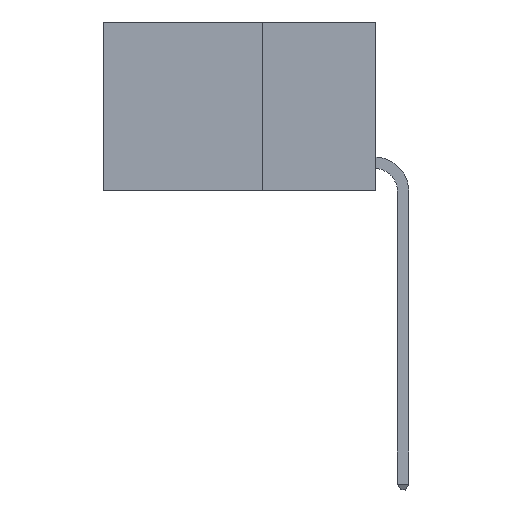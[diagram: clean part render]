
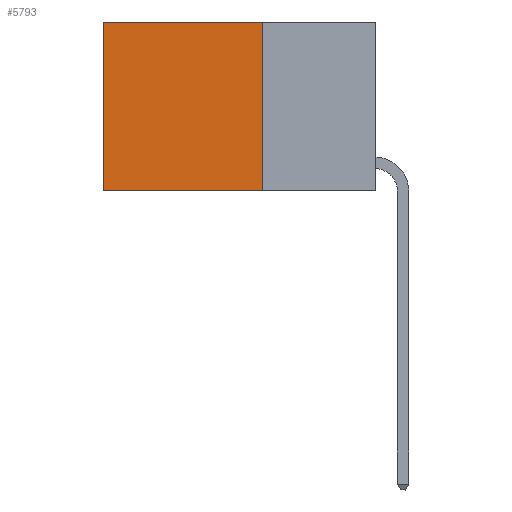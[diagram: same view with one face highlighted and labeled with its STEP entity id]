
A CAD part, left-side view. The second image highlights one B-rep face of the part: STEP entity #5793.
In plain terms, the highlighted planar face has unit normal (-1, 0, 0).
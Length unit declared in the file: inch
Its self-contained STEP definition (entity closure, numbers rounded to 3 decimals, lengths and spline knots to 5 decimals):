
#1654 = DIRECTION ( 'NONE',  ( 1., 0., 0. ) ) ;
#2324 = VERTEX_POINT ( 'NONE', #18005 ) ;
#2935 = VECTOR ( 'NONE', #12799, 39.37008 ) ;
#3043 = CARTESIAN_POINT ( 'NONE',  ( 0.2625, 0.25, 0. ) ) ;
#3224 = VECTOR ( 'NONE', #13335, 39.37008 ) ;
#5793 = ADVANCED_FACE ( 'NONE', ( #10645 ), #13223, .F. ) ;
#7062 = EDGE_CURVE ( 'NONE', #20031, #13822, #12133, .T. ) ;
#7628 = ORIENTED_EDGE ( 'NONE', *, *, #7062, .T. ) ;
#8103 = LINE ( 'NONE', #14609, #2935 ) ;
#8305 = EDGE_CURVE ( 'NONE', #20031, #17705, #24687, .T. ) ;
#8434 = ORIENTED_EDGE ( 'NONE', *, *, #9219, .T. ) ;
#8855 = ORIENTED_EDGE ( 'NONE', *, *, #16244, .F. ) ;
#8932 = DIRECTION ( 'NONE',  ( 0., 0., -1. ) ) ;
#8996 = LINE ( 'NONE', #22740, #3224 ) ;
#9219 = EDGE_CURVE ( 'NONE', #13822, #2324, #8996, .T. ) ;
#10230 = VECTOR ( 'NONE', #8932, 39.37008 ) ;
#10645 = FACE_OUTER_BOUND ( 'NONE', #12396, .T. ) ;
#12133 = LINE ( 'NONE', #3043, #22196 ) ;
#12396 = EDGE_LOOP ( 'NONE', ( #8434, #8855, #18407, #7628 ) ) ;
#12799 = DIRECTION ( 'NONE',  ( 0., 1., 0. ) ) ;
#13223 = PLANE ( 'NONE',  #23253 ) ;
#13335 = DIRECTION ( 'NONE',  ( 0., 0., -1. ) ) ;
#13822 = VERTEX_POINT ( 'NONE', #23038 ) ;
#14609 = CARTESIAN_POINT ( 'NONE',  ( 0.2625, 0.25, -0.37 ) ) ;
#15143 = DIRECTION ( 'NONE',  ( 0., 0., -1. ) ) ;
#16244 = EDGE_CURVE ( 'NONE', #17705, #2324, #8103, .T. ) ;
#16461 = DIRECTION ( 'NONE',  ( 0., 1., 0. ) ) ;
#16910 = CARTESIAN_POINT ( 'NONE',  ( 0.2625, 0.25, 0. ) ) ;
#17705 = VERTEX_POINT ( 'NONE', #21073 ) ;
#18005 = CARTESIAN_POINT ( 'NONE',  ( 0.2625, 0.6, -0.37 ) ) ;
#18407 = ORIENTED_EDGE ( 'NONE', *, *, #8305, .F. ) ;
#20031 = VERTEX_POINT ( 'NONE', #22853 ) ;
#20331 = CARTESIAN_POINT ( 'NONE',  ( 0.2625, 0.25, 0. ) ) ;
#21073 = CARTESIAN_POINT ( 'NONE',  ( 0.2625, 0.25, -0.37 ) ) ;
#22196 = VECTOR ( 'NONE', #16461, 39.37008 ) ;
#22740 = CARTESIAN_POINT ( 'NONE',  ( 0.2625, 0.6, 0. ) ) ;
#22853 = CARTESIAN_POINT ( 'NONE',  ( 0.2625, 0.25, 0. ) ) ;
#23038 = CARTESIAN_POINT ( 'NONE',  ( 0.2625, 0.6, 0. ) ) ;
#23253 = AXIS2_PLACEMENT_3D ( 'NONE', #16910, #1654, #15143 ) ;
#24687 = LINE ( 'NONE', #20331, #10230 ) ;
